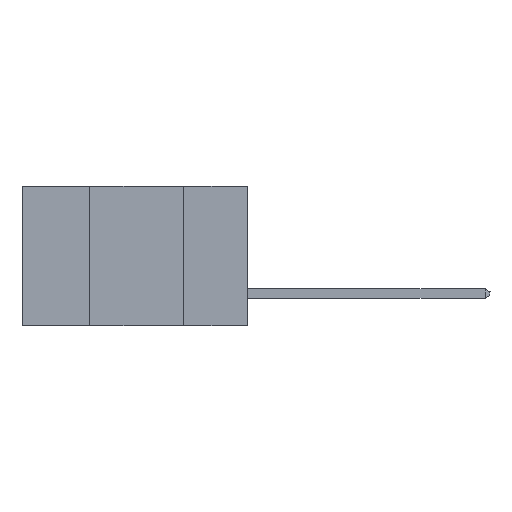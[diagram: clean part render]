
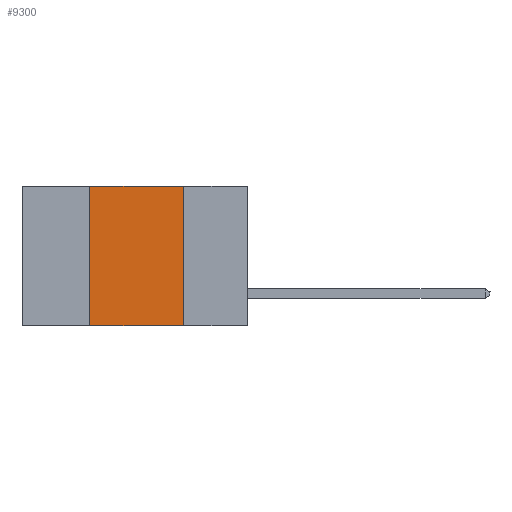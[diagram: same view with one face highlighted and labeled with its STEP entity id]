
A CAD part, left-side view. The second image highlights one B-rep face of the part: STEP entity #9300.
In plain terms, the highlighted planar face has unit normal (-1, 0, 0).
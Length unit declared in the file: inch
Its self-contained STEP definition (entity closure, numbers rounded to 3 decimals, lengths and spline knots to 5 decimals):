
#282 = EDGE_CURVE ( 'NONE', #13638, #14127, #8659, .T. ) ;
#913 = DIRECTION ( 'NONE',  ( 1., 0., 0. ) ) ;
#2326 = LINE ( 'NONE', #14889, #3518 ) ;
#2943 = VECTOR ( 'NONE', #22451, 39.37008 ) ;
#3518 = VECTOR ( 'NONE', #9689, 39.37008 ) ;
#4185 = DIRECTION ( 'NONE',  ( 0., -1., 0. ) ) ;
#4697 = CARTESIAN_POINT ( 'NONE',  ( 0., 0.17, -0.37 ) ) ;
#4951 = PLANE ( 'NONE',  #8158 ) ;
#5918 = ORIENTED_EDGE ( 'NONE', *, *, #8290, .F. ) ;
#6461 = CARTESIAN_POINT ( 'NONE',  ( 0., 0.42, -0.37 ) ) ;
#6648 = VERTEX_POINT ( 'NONE', #4697 ) ;
#6778 = ORIENTED_EDGE ( 'NONE', *, *, #282, .F. ) ;
#7189 = CARTESIAN_POINT ( 'NONE',  ( 0., 0.6, 0. ) ) ;
#7821 = VECTOR ( 'NONE', #4185, 39.37008 ) ;
#8158 = AXIS2_PLACEMENT_3D ( 'NONE', #19108, #913, #10313 ) ;
#8290 = EDGE_CURVE ( 'NONE', #18583, #6648, #2326, .T. ) ;
#8659 = LINE ( 'NONE', #6461, #17348 ) ;
#9060 = CARTESIAN_POINT ( 'NONE',  ( 0., 0.42, 0. ) ) ;
#9300 = ADVANCED_FACE ( 'NONE', ( #10428 ), #4951, .F. ) ;
#9689 = DIRECTION ( 'NONE',  ( 0., 0., -1. ) ) ;
#10313 = DIRECTION ( 'NONE',  ( 0., 0., -1. ) ) ;
#10428 = FACE_OUTER_BOUND ( 'NONE', #20437, .T. ) ;
#10864 = LINE ( 'NONE', #7189, #7821 ) ;
#10865 = EDGE_CURVE ( 'NONE', #13638, #6648, #14980, .T. ) ;
#11546 = CARTESIAN_POINT ( 'NONE',  ( 0., 0.42, -0.37 ) ) ;
#12075 = EDGE_CURVE ( 'NONE', #14127, #18583, #10864, .T. ) ;
#13638 = VERTEX_POINT ( 'NONE', #11546 ) ;
#14127 = VERTEX_POINT ( 'NONE', #9060 ) ;
#14889 = CARTESIAN_POINT ( 'NONE',  ( 0., 0.17, -0.37 ) ) ;
#14980 = LINE ( 'NONE', #22089, #2943 ) ;
#15689 = DIRECTION ( 'NONE',  ( 0., 0., 1. ) ) ;
#17348 = VECTOR ( 'NONE', #15689, 39.37008 ) ;
#17766 = ORIENTED_EDGE ( 'NONE', *, *, #12075, .F. ) ;
#18583 = VERTEX_POINT ( 'NONE', #22513 ) ;
#19108 = CARTESIAN_POINT ( 'NONE',  ( 0., 0.6, 0. ) ) ;
#19410 = ORIENTED_EDGE ( 'NONE', *, *, #10865, .T. ) ;
#20437 = EDGE_LOOP ( 'NONE', ( #5918, #17766, #6778, #19410 ) ) ;
#22089 = CARTESIAN_POINT ( 'NONE',  ( 0., 0.6, -0.37 ) ) ;
#22451 = DIRECTION ( 'NONE',  ( 0., -1., 0. ) ) ;
#22513 = CARTESIAN_POINT ( 'NONE',  ( 0., 0.17, 0. ) ) ;
